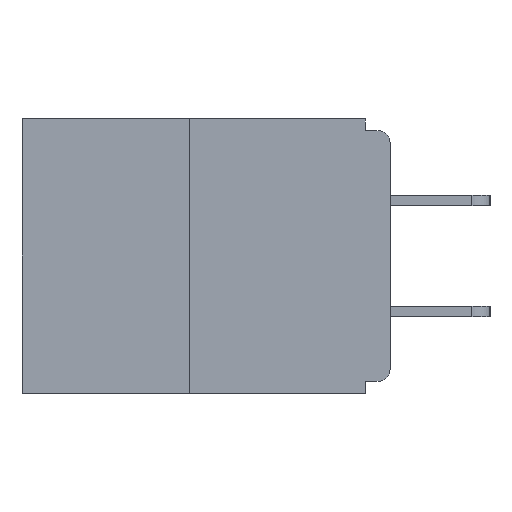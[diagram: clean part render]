
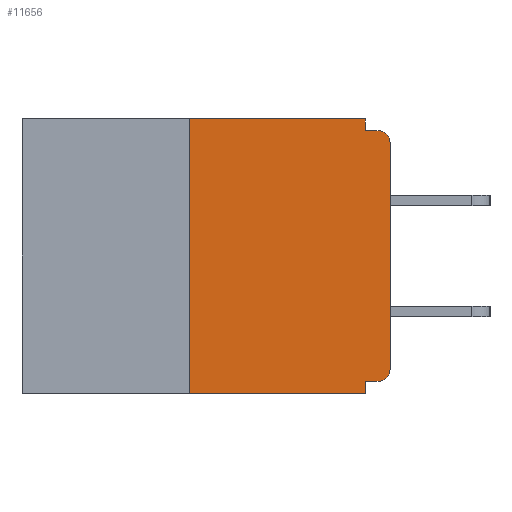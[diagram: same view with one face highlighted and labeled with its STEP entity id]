
A CAD part, left-side view. The second image highlights one B-rep face of the part: STEP entity #11656.
In plain terms, the highlighted planar face has unit normal (-1, 0, 0).
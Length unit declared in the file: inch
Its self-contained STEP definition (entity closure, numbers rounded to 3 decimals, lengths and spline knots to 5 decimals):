
#40 = LINE ( 'NONE', #3706, #6770 ) ;
#258 = EDGE_CURVE ( 'NONE', #2555, #4907, #2632, .T. ) ;
#385 = CARTESIAN_POINT ( 'NONE',  ( 0., 0.031, -0.343 ) ) ;
#607 = CARTESIAN_POINT ( 'NONE',  ( 0., 0.031, 0. ) ) ;
#734 = EDGE_CURVE ( 'NONE', #9127, #4120, #8391, .T. ) ;
#797 = ORIENTED_EDGE ( 'NONE', *, *, #5636, .T. ) ;
#1536 = AXIS2_PLACEMENT_3D ( 'NONE', #5875, #1749, #11748 ) ;
#1637 = CARTESIAN_POINT ( 'NONE',  ( 0., 0., -0.313 ) ) ;
#1705 = LINE ( 'NONE', #2040, #12460 ) ;
#1719 = ORIENTED_EDGE ( 'NONE', *, *, #4482, .T. ) ;
#1749 = DIRECTION ( 'NONE',  ( -1., 0., 0. ) ) ;
#2040 = CARTESIAN_POINT ( 'NONE',  ( 0., 0., -0.015 ) ) ;
#2243 = CARTESIAN_POINT ( 'NONE',  ( 0., 0.25, -0.343 ) ) ;
#2301 = ORIENTED_EDGE ( 'NONE', *, *, #258, .T. ) ;
#2361 = AXIS2_PLACEMENT_3D ( 'NONE', #12327, #3457, #9383 ) ;
#2555 = VERTEX_POINT ( 'NONE', #1637 ) ;
#2632 = LINE ( 'NONE', #9925, #10886 ) ;
#3009 = LINE ( 'NONE', #12025, #3639 ) ;
#3457 = DIRECTION ( 'NONE',  ( -1., 0., 0. ) ) ;
#3512 = ORIENTED_EDGE ( 'NONE', *, *, #734, .F. ) ;
#3639 = VECTOR ( 'NONE', #6053, 39.37008 ) ;
#3706 = CARTESIAN_POINT ( 'NONE',  ( 0., 0., -0.328 ) ) ;
#3757 = DIRECTION ( 'NONE',  ( 0., 0., -1. ) ) ;
#3855 = ORIENTED_EDGE ( 'NONE', *, *, #10452, .F. ) ;
#3913 = ORIENTED_EDGE ( 'NONE', *, *, #3999, .F. ) ;
#3999 = EDGE_CURVE ( 'NONE', #5581, #5288, #3009, .T. ) ;
#4120 = VERTEX_POINT ( 'NONE', #385 ) ;
#4389 = ORIENTED_EDGE ( 'NONE', *, *, #8738, .F. ) ;
#4482 = EDGE_CURVE ( 'NONE', #5581, #4120, #11100, .T. ) ;
#4737 = CARTESIAN_POINT ( 'NONE',  ( 0., 0.46, 0. ) ) ;
#4907 = VERTEX_POINT ( 'NONE', #10821 ) ;
#4913 = DIRECTION ( 'NONE',  ( 0., -1., 0. ) ) ;
#4939 = DIRECTION ( 'NONE',  ( 0., 0., -1. ) ) ;
#5095 = VECTOR ( 'NONE', #4913, 39.37008 ) ;
#5288 = VERTEX_POINT ( 'NONE', #10566 ) ;
#5560 = DIRECTION ( 'NONE',  ( 0., 0., -1. ) ) ;
#5581 = VERTEX_POINT ( 'NONE', #2243 ) ;
#5587 = CARTESIAN_POINT ( 'NONE',  ( 0., 0.031, -0.328 ) ) ;
#5636 = EDGE_CURVE ( 'NONE', #8021, #2555, #7023, .T. ) ;
#5875 = CARTESIAN_POINT ( 'NONE',  ( 0., 0.015, -0.03 ) ) ;
#5988 = CARTESIAN_POINT ( 'NONE',  ( 0., 0.46, -0.343 ) ) ;
#6022 = LINE ( 'NONE', #4737, #5095 ) ;
#6036 = DIRECTION ( 'NONE',  ( 0., -1., 0. ) ) ;
#6053 = DIRECTION ( 'NONE',  ( 0., 0., 1. ) ) ;
#6138 = DIRECTION ( 'NONE',  ( 0., -1., 0. ) ) ;
#6220 = VECTOR ( 'NONE', #5560, 39.37008 ) ;
#6534 = EDGE_CURVE ( 'NONE', #10408, #11159, #10284, .T. ) ;
#6572 = ORIENTED_EDGE ( 'NONE', *, *, #8694, .T. ) ;
#6770 = VECTOR ( 'NONE', #7847, 39.37008 ) ;
#6909 = CARTESIAN_POINT ( 'NONE',  ( 0., 0.031, -0.343 ) ) ;
#7003 = EDGE_CURVE ( 'NONE', #11159, #8438, #1705, .T. ) ;
#7023 = CIRCLE ( 'NONE', #2361, 0.015 ) ;
#7847 = DIRECTION ( 'NONE',  ( 0., 1., 0. ) ) ;
#7861 = CARTESIAN_POINT ( 'NONE',  ( 0., 0.46, 0. ) ) ;
#8021 = VERTEX_POINT ( 'NONE', #8462 ) ;
#8391 = LINE ( 'NONE', #6909, #12587 ) ;
#8438 = VERTEX_POINT ( 'NONE', #8458 ) ;
#8458 = CARTESIAN_POINT ( 'NONE',  ( 0., 0.015, -0.015 ) ) ;
#8459 = VECTOR ( 'NONE', #6036, 39.37008 ) ;
#8462 = CARTESIAN_POINT ( 'NONE',  ( 0., 0.015, -0.328 ) ) ;
#8649 = ORIENTED_EDGE ( 'NONE', *, *, #7003, .F. ) ;
#8694 = EDGE_CURVE ( 'NONE', #4907, #8438, #12721, .T. ) ;
#8738 = EDGE_CURVE ( 'NONE', #5288, #10408, #6022, .T. ) ;
#9127 = VERTEX_POINT ( 'NONE', #5587 ) ;
#9383 = DIRECTION ( 'NONE',  ( 0., 0., -1. ) ) ;
#9499 = AXIS2_PLACEMENT_3D ( 'NONE', #7861, #12856, #3757 ) ;
#9870 = ORIENTED_EDGE ( 'NONE', *, *, #6534, .F. ) ;
#9925 = CARTESIAN_POINT ( 'NONE',  ( 0., 0., 0. ) ) ;
#9994 = FACE_OUTER_BOUND ( 'NONE', #10598, .T. ) ;
#10284 = LINE ( 'NONE', #12601, #6220 ) ;
#10408 = VERTEX_POINT ( 'NONE', #607 ) ;
#10452 = EDGE_CURVE ( 'NONE', #8021, #9127, #40, .T. ) ;
#10566 = CARTESIAN_POINT ( 'NONE',  ( 0., 0.25, 0. ) ) ;
#10598 = EDGE_LOOP ( 'NONE', ( #4389, #3913, #1719, #3512, #3855, #797, #2301, #6572, #8649, #9870 ) ) ;
#10813 = PLANE ( 'NONE',  #9499 ) ;
#10821 = CARTESIAN_POINT ( 'NONE',  ( 0., 0., -0.03 ) ) ;
#10886 = VECTOR ( 'NONE', #12910, 39.37008 ) ;
#11100 = LINE ( 'NONE', #5988, #8459 ) ;
#11159 = VERTEX_POINT ( 'NONE', #11822 ) ;
#11656 = ADVANCED_FACE ( 'NONE', ( #9994 ), #10813, .F. ) ;
#11748 = DIRECTION ( 'NONE',  ( 0., 0., -1. ) ) ;
#11822 = CARTESIAN_POINT ( 'NONE',  ( 0., 0.031, -0.015 ) ) ;
#12025 = CARTESIAN_POINT ( 'NONE',  ( 0., 0.25, 0. ) ) ;
#12327 = CARTESIAN_POINT ( 'NONE',  ( 0., 0.015, -0.313 ) ) ;
#12460 = VECTOR ( 'NONE', #6138, 39.37008 ) ;
#12587 = VECTOR ( 'NONE', #4939, 39.37008 ) ;
#12601 = CARTESIAN_POINT ( 'NONE',  ( 0., 0.031, 0. ) ) ;
#12721 = CIRCLE ( 'NONE', #1536, 0.015 ) ;
#12856 = DIRECTION ( 'NONE',  ( 1., 0., 0. ) ) ;
#12910 = DIRECTION ( 'NONE',  ( 0., 0., 1. ) ) ;
